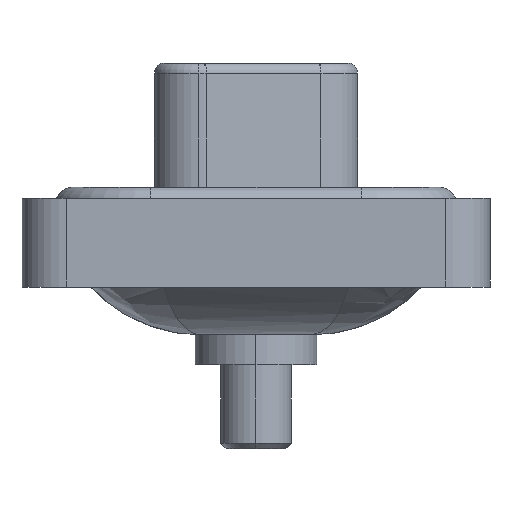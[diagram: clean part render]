
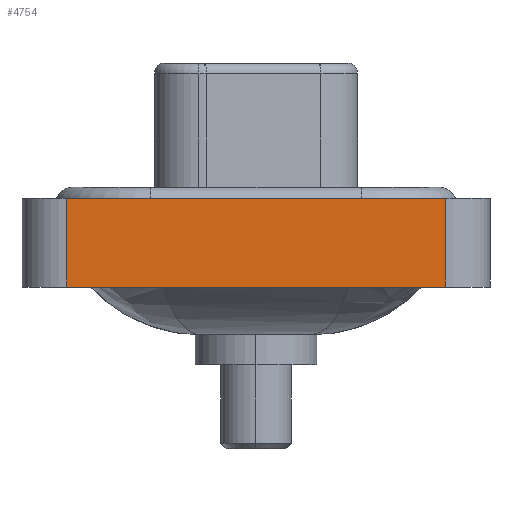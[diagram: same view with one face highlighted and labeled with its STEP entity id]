
A CAD part, left-side view. The second image highlights one B-rep face of the part: STEP entity #4754.
In plain terms, the highlighted planar face has unit normal (-1, 0, 0).
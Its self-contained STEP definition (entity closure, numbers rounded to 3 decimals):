
#45 = VECTOR ( 'NONE', #6059, 1000. ) ;
#47 = ORIENTED_EDGE ( 'NONE', *, *, #17809, .F. ) ;
#2259 = EDGE_LOOP ( 'NONE', ( #10111, #8101, #47, #10399 ) ) ;
#4319 = VECTOR ( 'NONE', #5426, 1000. ) ;
#4460 = CARTESIAN_POINT ( 'NONE',  ( -7.35, -8.55, 0.4 ) ) ;
#4754 = ADVANCED_FACE ( 'NONE', ( #13018 ), #6034, .T. ) ;
#5426 = DIRECTION ( 'NONE',  ( 0., -1., 0. ) ) ;
#6034 = PLANE ( 'NONE',  #10268 ) ;
#6059 = DIRECTION ( 'NONE',  ( 0., -1., 0. ) ) ;
#7008 = VERTEX_POINT ( 'NONE', #14451 ) ;
#7120 = CARTESIAN_POINT ( 'NONE',  ( -7.35, -8.55, -3.6 ) ) ;
#7671 = LINE ( 'NONE', #8879, #10094 ) ;
#8101 = ORIENTED_EDGE ( 'NONE', *, *, #17063, .F. ) ;
#8712 = VECTOR ( 'NONE', #16458, 1000. ) ;
#8879 = CARTESIAN_POINT ( 'NONE',  ( -7.35, 8.55, -3.6 ) ) ;
#9153 = DIRECTION ( 'NONE',  ( 0., 0., 1. ) ) ;
#9557 = CARTESIAN_POINT ( 'NONE',  ( -7.35, -8.55, 0.4 ) ) ;
#9968 = DIRECTION ( 'NONE',  ( -1., 0., 0. ) ) ;
#10094 = VECTOR ( 'NONE', #9153, 1000. ) ;
#10111 = ORIENTED_EDGE ( 'NONE', *, *, #17074, .T. ) ;
#10268 = AXIS2_PLACEMENT_3D ( 'NONE', #7120, #9968, #12747 ) ;
#10399 = ORIENTED_EDGE ( 'NONE', *, *, #13749, .T. ) ;
#10814 = CARTESIAN_POINT ( 'NONE',  ( -7.35, -8.55, -3.6 ) ) ;
#10839 = LINE ( 'NONE', #15188, #8712 ) ;
#11666 = CARTESIAN_POINT ( 'NONE',  ( -7.35, -8.55, -3.6 ) ) ;
#12747 = DIRECTION ( 'NONE',  ( 0., 0., 1. ) ) ;
#13018 = FACE_OUTER_BOUND ( 'NONE', #2259, .T. ) ;
#13031 = CARTESIAN_POINT ( 'NONE',  ( -7.35, 8.55, 0.4 ) ) ;
#13749 = EDGE_CURVE ( 'NONE', #7008, #16169, #17092, .T. ) ;
#14390 = VERTEX_POINT ( 'NONE', #13031 ) ;
#14451 = CARTESIAN_POINT ( 'NONE',  ( -7.35, 8.55, -3.6 ) ) ;
#15188 = CARTESIAN_POINT ( 'NONE',  ( -7.35, -8.55, -3.6 ) ) ;
#16169 = VERTEX_POINT ( 'NONE', #10814 ) ;
#16371 = LINE ( 'NONE', #9557, #4319 ) ;
#16458 = DIRECTION ( 'NONE',  ( 0., 0., 1. ) ) ;
#17063 = EDGE_CURVE ( 'NONE', #14390, #18082, #16371, .T. ) ;
#17074 = EDGE_CURVE ( 'NONE', #16169, #18082, #10839, .T. ) ;
#17092 = LINE ( 'NONE', #11666, #45 ) ;
#17809 = EDGE_CURVE ( 'NONE', #7008, #14390, #7671, .T. ) ;
#18082 = VERTEX_POINT ( 'NONE', #4460 ) ;
